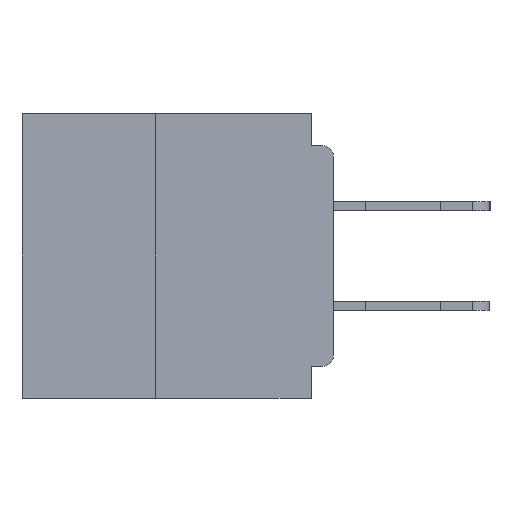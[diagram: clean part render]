
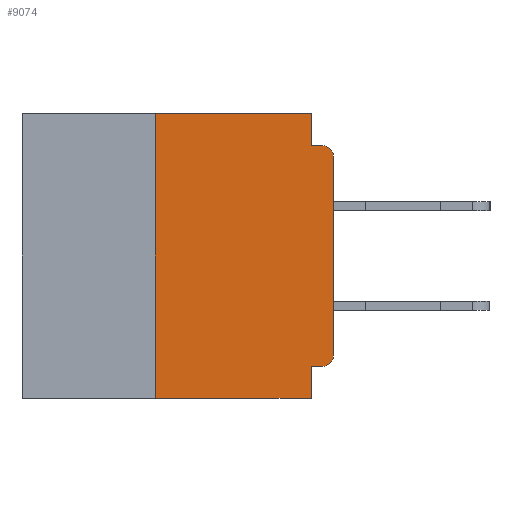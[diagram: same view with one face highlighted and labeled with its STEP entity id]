
A CAD part, left-side view. The second image highlights one B-rep face of the part: STEP entity #9074.
In plain terms, the highlighted planar face has unit normal (-1, 0, 0).
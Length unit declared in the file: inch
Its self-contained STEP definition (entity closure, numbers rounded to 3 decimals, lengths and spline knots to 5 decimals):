
#446 = ORIENTED_EDGE ( 'NONE', *, *, #16160, .T. ) ;
#1032 = EDGE_CURVE ( 'NONE', #8816, #6129, #29169, .T. ) ;
#1835 = VECTOR ( 'NONE', #14479, 39.37008 ) ;
#2821 = CARTESIAN_POINT ( 'NONE',  ( 0., 0.437, 0. ) ) ;
#3580 = ORIENTED_EDGE ( 'NONE', *, *, #5857, .F. ) ;
#3767 = DIRECTION ( 'NONE',  ( 0., 0., -1. ) ) ;
#5736 = ORIENTED_EDGE ( 'NONE', *, *, #29631, .T. ) ;
#5821 = CARTESIAN_POINT ( 'NONE',  ( 0., 0.25, -0.4 ) ) ;
#5857 = EDGE_CURVE ( 'NONE', #14399, #9807, #17788, .T. ) ;
#5900 = CARTESIAN_POINT ( 'NONE',  ( 0., 0.437, 0. ) ) ;
#5941 = EDGE_CURVE ( 'NONE', #28845, #8816, #14308, .T. ) ;
#6129 = VERTEX_POINT ( 'NONE', #43798 ) ;
#6628 = VECTOR ( 'NONE', #18151, 39.37008 ) ;
#6790 = VECTOR ( 'NONE', #31716, 39.37008 ) ;
#7751 = DIRECTION ( 'NONE',  ( 0., 0., 1. ) ) ;
#8816 = VERTEX_POINT ( 'NONE', #12636 ) ;
#9074 = ADVANCED_FACE ( 'NONE', ( #10514 ), #25204, .F. ) ;
#9287 = ORIENTED_EDGE ( 'NONE', *, *, #5941, .F. ) ;
#9748 = EDGE_CURVE ( 'NONE', #48015, #38440, #21548, .T. ) ;
#9807 = VERTEX_POINT ( 'NONE', #22202 ) ;
#10514 = FACE_OUTER_BOUND ( 'NONE', #42206, .T. ) ;
#11118 = AXIS2_PLACEMENT_3D ( 'NONE', #14694, #40522, #18391 ) ;
#11966 = DIRECTION ( 'NONE',  ( 0., -1., 0. ) ) ;
#12559 = LINE ( 'NONE', #26162, #31082 ) ;
#12596 = CARTESIAN_POINT ( 'NONE',  ( 0., 0.031, -0.045 ) ) ;
#12636 = CARTESIAN_POINT ( 'NONE',  ( 0., 0.25, 0. ) ) ;
#12808 = CARTESIAN_POINT ( 'NONE',  ( 0., 0., -0.355 ) ) ;
#13235 = ORIENTED_EDGE ( 'NONE', *, *, #9748, .F. ) ;
#13420 = CARTESIAN_POINT ( 'NONE',  ( 0., 0.437, -0.4 ) ) ;
#14308 = LINE ( 'NONE', #5821, #6790 ) ;
#14399 = VERTEX_POINT ( 'NONE', #30509 ) ;
#14479 = DIRECTION ( 'NONE',  ( 0., -1., 0. ) ) ;
#14600 = CARTESIAN_POINT ( 'NONE',  ( 0., 0.25, -0.4 ) ) ;
#14694 = CARTESIAN_POINT ( 'NONE',  ( 0., 0.015, -0.06 ) ) ;
#15039 = VERTEX_POINT ( 'NONE', #15888 ) ;
#15631 = DIRECTION ( 'NONE',  ( -1., 0., 0. ) ) ;
#15888 = CARTESIAN_POINT ( 'NONE',  ( 0., 0., -0.34 ) ) ;
#15965 = LINE ( 'NONE', #25954, #47727 ) ;
#16160 = EDGE_CURVE ( 'NONE', #14399, #15039, #47780, .T. ) ;
#16525 = DIRECTION ( 'NONE',  ( 0., 1., 0. ) ) ;
#17788 = LINE ( 'NONE', #12808, #36319 ) ;
#17934 = DIRECTION ( 'NONE',  ( 1., 0., 0. ) ) ;
#18151 = DIRECTION ( 'NONE',  ( 0., 0., -1. ) ) ;
#18391 = DIRECTION ( 'NONE',  ( 0., 0., -1. ) ) ;
#19320 = VECTOR ( 'NONE', #11966, 39.37008 ) ;
#21079 = VERTEX_POINT ( 'NONE', #27287 ) ;
#21536 = VERTEX_POINT ( 'NONE', #44850 ) ;
#21548 = LINE ( 'NONE', #40325, #1835 ) ;
#22202 = CARTESIAN_POINT ( 'NONE',  ( 0., 0.031, -0.355 ) ) ;
#24404 = ORIENTED_EDGE ( 'NONE', *, *, #34615, .T. ) ;
#25204 = PLANE ( 'NONE',  #27507 ) ;
#25356 = EDGE_CURVE ( 'NONE', #9807, #21079, #15965, .T. ) ;
#25954 = CARTESIAN_POINT ( 'NONE',  ( 0., 0.031, -0.4 ) ) ;
#25996 = EDGE_CURVE ( 'NONE', #6129, #48015, #45933, .T. ) ;
#26162 = CARTESIAN_POINT ( 'NONE',  ( 0., 0., 0. ) ) ;
#26256 = VECTOR ( 'NONE', #39261, 39.37008 ) ;
#26479 = EDGE_CURVE ( 'NONE', #28845, #21079, #45888, .T. ) ;
#27287 = CARTESIAN_POINT ( 'NONE',  ( 0., 0.031, -0.4 ) ) ;
#27507 = AXIS2_PLACEMENT_3D ( 'NONE', #2821, #17934, #43786 ) ;
#28845 = VERTEX_POINT ( 'NONE', #14600 ) ;
#28887 = ORIENTED_EDGE ( 'NONE', *, *, #25996, .F. ) ;
#29169 = LINE ( 'NONE', #5900, #19320 ) ;
#29631 = EDGE_CURVE ( 'NONE', #15039, #21536, #12559, .T. ) ;
#30509 = CARTESIAN_POINT ( 'NONE',  ( 0., 0.015, -0.355 ) ) ;
#31082 = VECTOR ( 'NONE', #7751, 39.37008 ) ;
#31716 = DIRECTION ( 'NONE',  ( 0., 0., 1. ) ) ;
#33792 = CIRCLE ( 'NONE', #11118, 0.015 ) ;
#34615 = EDGE_CURVE ( 'NONE', #21536, #38440, #33792, .T. ) ;
#36319 = VECTOR ( 'NONE', #16525, 39.37008 ) ;
#36592 = CARTESIAN_POINT ( 'NONE',  ( 0., 0.031, 0. ) ) ;
#37805 = CARTESIAN_POINT ( 'NONE',  ( 0., 0.015, -0.34 ) ) ;
#38085 = ORIENTED_EDGE ( 'NONE', *, *, #1032, .F. ) ;
#38440 = VERTEX_POINT ( 'NONE', #42452 ) ;
#39261 = DIRECTION ( 'NONE',  ( 0., -1., 0. ) ) ;
#40325 = CARTESIAN_POINT ( 'NONE',  ( 0., 0., -0.045 ) ) ;
#40522 = DIRECTION ( 'NONE',  ( -1., 0., 0. ) ) ;
#41473 = DIRECTION ( 'NONE',  ( 0., 0., -1. ) ) ;
#42206 = EDGE_LOOP ( 'NONE', ( #5736, #24404, #13235, #28887, #38085, #9287, #45694, #47532, #3580, #446 ) ) ;
#42452 = CARTESIAN_POINT ( 'NONE',  ( 0., 0.015, -0.045 ) ) ;
#43221 = AXIS2_PLACEMENT_3D ( 'NONE', #37805, #15631, #41473 ) ;
#43786 = DIRECTION ( 'NONE',  ( 0., 0., -1. ) ) ;
#43798 = CARTESIAN_POINT ( 'NONE',  ( 0., 0.031, 0. ) ) ;
#44850 = CARTESIAN_POINT ( 'NONE',  ( 0., 0., -0.06 ) ) ;
#45694 = ORIENTED_EDGE ( 'NONE', *, *, #26479, .T. ) ;
#45888 = LINE ( 'NONE', #13420, #26256 ) ;
#45933 = LINE ( 'NONE', #36592, #6628 ) ;
#47532 = ORIENTED_EDGE ( 'NONE', *, *, #25356, .F. ) ;
#47727 = VECTOR ( 'NONE', #3767, 39.37008 ) ;
#47780 = CIRCLE ( 'NONE', #43221, 0.015 ) ;
#48015 = VERTEX_POINT ( 'NONE', #12596 ) ;
